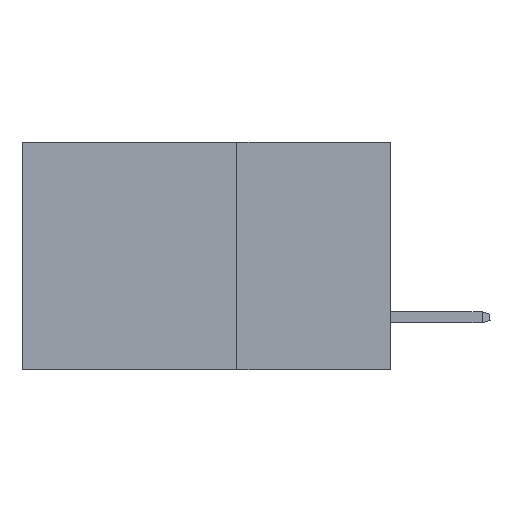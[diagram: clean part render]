
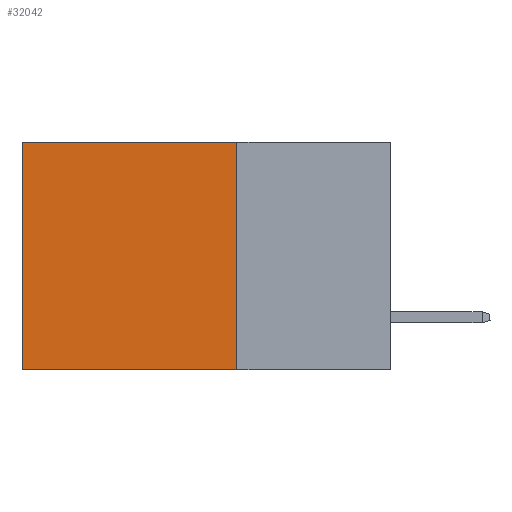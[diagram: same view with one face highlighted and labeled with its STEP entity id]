
A CAD part, left-side view. The second image highlights one B-rep face of the part: STEP entity #32042.
In plain terms, the highlighted planar face has unit normal (-1, 0, 0).
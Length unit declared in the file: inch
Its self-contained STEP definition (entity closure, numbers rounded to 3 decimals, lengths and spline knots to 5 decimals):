
#144 = EDGE_CURVE ( 'NONE', #45703, #28928, #34109, .T. ) ;
#714 = VECTOR ( 'NONE', #30596, 39.37008 ) ;
#5227 = ORIENTED_EDGE ( 'NONE', *, *, #13852, .T. ) ;
#5931 = FACE_OUTER_BOUND ( 'NONE', #41262, .T. ) ;
#6869 = CARTESIAN_POINT ( 'NONE',  ( 0.2875, 0.25, 0. ) ) ;
#7361 = VECTOR ( 'NONE', #32340, 39.37008 ) ;
#8016 = VECTOR ( 'NONE', #35510, 39.37008 ) ;
#9566 = DIRECTION ( 'NONE',  ( 1., 0., 0. ) ) ;
#9661 = ORIENTED_EDGE ( 'NONE', *, *, #14319, .F. ) ;
#13852 = EDGE_CURVE ( 'NONE', #45703, #22832, #34243, .T. ) ;
#14319 = EDGE_CURVE ( 'NONE', #28928, #37169, #17784, .T. ) ;
#14824 = VECTOR ( 'NONE', #18897, 39.37008 ) ;
#15086 = CARTESIAN_POINT ( 'NONE',  ( 0.2875, 0.25, 0. ) ) ;
#16765 = PLANE ( 'NONE',  #20333 ) ;
#17784 = LINE ( 'NONE', #31542, #8016 ) ;
#18897 = DIRECTION ( 'NONE',  ( 0., 1., 0. ) ) ;
#20215 = EDGE_CURVE ( 'NONE', #22832, #37169, #36649, .T. ) ;
#20333 = AXIS2_PLACEMENT_3D ( 'NONE', #41875, #9566, #38200 ) ;
#22832 = VERTEX_POINT ( 'NONE', #33229 ) ;
#23941 = CARTESIAN_POINT ( 'NONE',  ( 0.2875, 0.6, -0.37 ) ) ;
#26964 = CARTESIAN_POINT ( 'NONE',  ( 0.2875, 0.6, 0. ) ) ;
#28928 = VERTEX_POINT ( 'NONE', #47084 ) ;
#29692 = ORIENTED_EDGE ( 'NONE', *, *, #144, .F. ) ;
#30596 = DIRECTION ( 'NONE',  ( 0., 0., -1. ) ) ;
#31542 = CARTESIAN_POINT ( 'NONE',  ( 0.2875, 0.25, -0.37 ) ) ;
#32042 = ADVANCED_FACE ( 'NONE', ( #5931 ), #16765, .F. ) ;
#32065 = ORIENTED_EDGE ( 'NONE', *, *, #20215, .T. ) ;
#32340 = DIRECTION ( 'NONE',  ( 0., 0., -1. ) ) ;
#33229 = CARTESIAN_POINT ( 'NONE',  ( 0.2875, 0.6, 0. ) ) ;
#34109 = LINE ( 'NONE', #6869, #7361 ) ;
#34243 = LINE ( 'NONE', #40667, #14824 ) ;
#35510 = DIRECTION ( 'NONE',  ( 0., 1., 0. ) ) ;
#36649 = LINE ( 'NONE', #26964, #714 ) ;
#37169 = VERTEX_POINT ( 'NONE', #23941 ) ;
#38200 = DIRECTION ( 'NONE',  ( 0., 0., -1. ) ) ;
#40667 = CARTESIAN_POINT ( 'NONE',  ( 0.2875, 0.25, 0. ) ) ;
#41262 = EDGE_LOOP ( 'NONE', ( #32065, #9661, #29692, #5227 ) ) ;
#41875 = CARTESIAN_POINT ( 'NONE',  ( 0.2875, 0.25, 0. ) ) ;
#45703 = VERTEX_POINT ( 'NONE', #15086 ) ;
#47084 = CARTESIAN_POINT ( 'NONE',  ( 0.2875, 0.25, -0.37 ) ) ;
